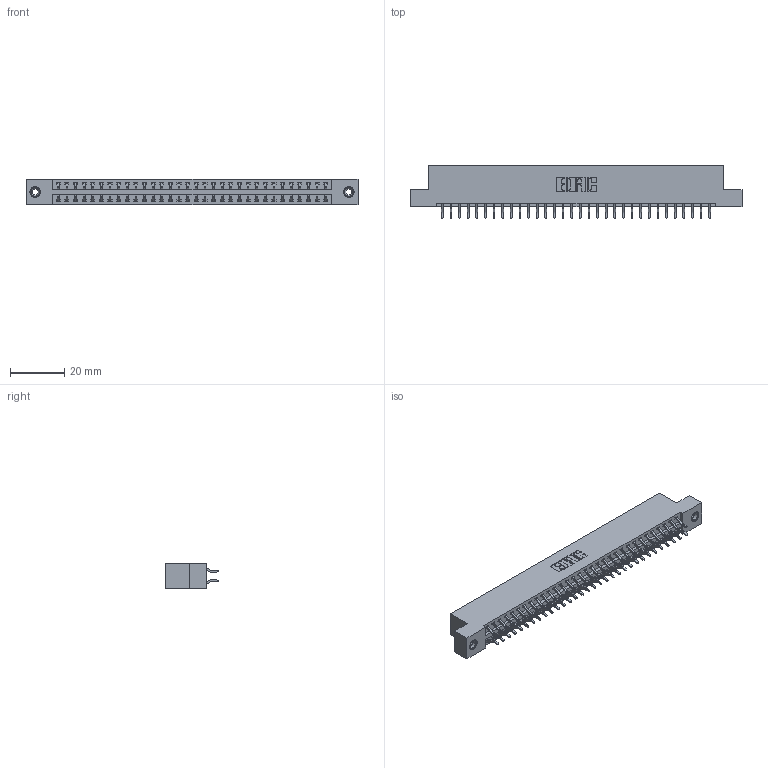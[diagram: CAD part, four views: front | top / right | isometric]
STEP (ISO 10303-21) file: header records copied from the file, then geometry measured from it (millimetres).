
FILE_DESCRIPTION (( 'STEP AP203' ), '1' );
FILE_NAME ('396-064-556-208.STEP', '2018-09-08T17:39:41', ( '' ), ( '' ), 'SwSTEP 2.0', 'SolidWorks 2016', '' );
FILE_SCHEMA (( 'CONFIG_CONTROL_DESIGN' ));
Length unit declared in the file: inch
Products named in the file (4): 346 Part_Flush Mounting Lugs - 0.156 Dia-TI; 345-292-001_556 Tail; 345-250-001_345-250-003-102; 396-064-556-208
Assembly tree (67 placements, depth 2):
  396-064-556-208
    346 Part_Flush Mounting Lugs - 0.156 Dia-TI
    345-292-001_556 Tail  x64
    345-250-001_345-250-003-102  x2
Bounding box: 122.17 x 19.57 x 9.4 mm (x, y, z)
Volume: 672.8 mm3; surface area: 15609.2 mm2
Topology: 66 solids, 67 shells, 3893 faces, 11537 edges, 7598 vertices
Faces by surface type: plane 2603, cylinder 1274, cone 12, torus 4
Entity records: 23636 total; most frequent: CARTESIAN_POINT 3907, ORIENTED_EDGE 3822, DIRECTION 3509, EDGE_CURVE 1911, VECTOR 1623, LINE 1623, VERTEX_POINT 1268, AXIS2_PLACEMENT_3D 943
